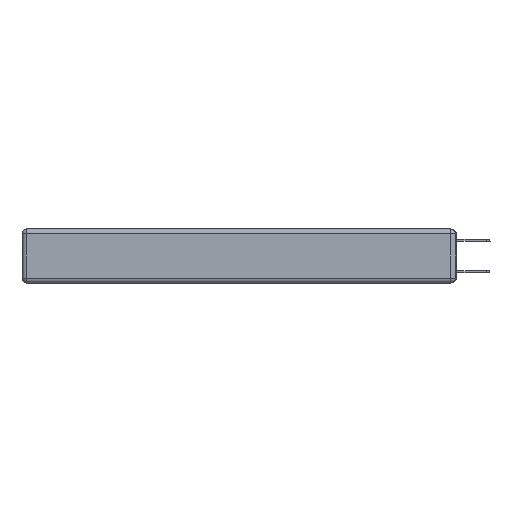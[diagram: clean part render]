
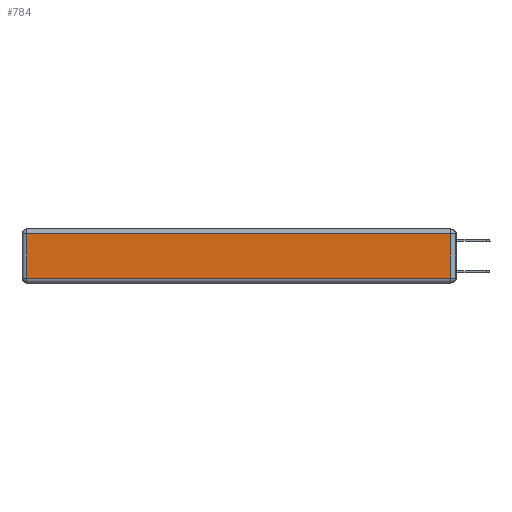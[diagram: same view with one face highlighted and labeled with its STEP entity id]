
A CAD part, left-side view. The second image highlights one B-rep face of the part: STEP entity #784.
In plain terms, the highlighted planar face has unit normal (-1, 0, 0).
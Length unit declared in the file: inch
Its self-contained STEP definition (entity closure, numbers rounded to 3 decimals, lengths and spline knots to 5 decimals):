
#784 = ADVANCED_FACE ( 'NONE', ( #7950 ), #14610, .T. ) ;
#2665 = CARTESIAN_POINT ( 'NONE',  ( 0., 2.72, -0.03 ) ) ;
#5371 = LINE ( 'NONE', #16975, #28543 ) ;
#6753 = DIRECTION ( 'NONE',  ( 0., 0., 1. ) ) ;
#6854 = VERTEX_POINT ( 'NONE', #11180 ) ;
#6976 = CARTESIAN_POINT ( 'NONE',  ( 0., 2.75, -0.03 ) ) ;
#7052 = ORIENTED_EDGE ( 'NONE', *, *, #9930, .T. ) ;
#7124 = LINE ( 'NONE', #6976, #26801 ) ;
#7950 = FACE_OUTER_BOUND ( 'NONE', #23447, .T. ) ;
#8433 = CARTESIAN_POINT ( 'NONE',  ( 0., 0.03, -0.313 ) ) ;
#9315 = ORIENTED_EDGE ( 'NONE', *, *, #19099, .T. ) ;
#9930 = EDGE_CURVE ( 'NONE', #11131, #17355, #5371, .T. ) ;
#10150 = DIRECTION ( 'NONE',  ( 0., 0., -1. ) ) ;
#11091 = ORIENTED_EDGE ( 'NONE', *, *, #26336, .T. ) ;
#11131 = VERTEX_POINT ( 'NONE', #2665 ) ;
#11180 = CARTESIAN_POINT ( 'NONE',  ( 0., 0.03, -0.03 ) ) ;
#12395 = AXIS2_PLACEMENT_3D ( 'NONE', #23473, #19423, #12870 ) ;
#12870 = DIRECTION ( 'NONE',  ( 0., 0., 1. ) ) ;
#13628 = DIRECTION ( 'NONE',  ( 0., 1., 0. ) ) ;
#14610 = PLANE ( 'NONE',  #12395 ) ;
#15661 = DIRECTION ( 'NONE',  ( 0., -1., 0. ) ) ;
#15860 = LINE ( 'NONE', #24742, #25571 ) ;
#15976 = CARTESIAN_POINT ( 'NONE',  ( 0., 2.72, -0.313 ) ) ;
#16975 = CARTESIAN_POINT ( 'NONE',  ( 0., 2.72, -0.343 ) ) ;
#17355 = VERTEX_POINT ( 'NONE', #15976 ) ;
#17975 = LINE ( 'NONE', #24398, #22885 ) ;
#19099 = EDGE_CURVE ( 'NONE', #6854, #11131, #7124, .T. ) ;
#19423 = DIRECTION ( 'NONE',  ( -1., 0., 0. ) ) ;
#22885 = VECTOR ( 'NONE', #15661, 39.37008 ) ;
#23447 = EDGE_LOOP ( 'NONE', ( #28520, #11091, #9315, #7052 ) ) ;
#23473 = CARTESIAN_POINT ( 'NONE',  ( 0., 0., -0.343 ) ) ;
#24398 = CARTESIAN_POINT ( 'NONE',  ( 0., 0., -0.313 ) ) ;
#24742 = CARTESIAN_POINT ( 'NONE',  ( 0., 0.03, -0.343 ) ) ;
#24755 = VERTEX_POINT ( 'NONE', #8433 ) ;
#25571 = VECTOR ( 'NONE', #6753, 39.37008 ) ;
#26336 = EDGE_CURVE ( 'NONE', #24755, #6854, #15860, .T. ) ;
#26655 = EDGE_CURVE ( 'NONE', #17355, #24755, #17975, .T. ) ;
#26801 = VECTOR ( 'NONE', #13628, 39.37008 ) ;
#28520 = ORIENTED_EDGE ( 'NONE', *, *, #26655, .T. ) ;
#28543 = VECTOR ( 'NONE', #10150, 39.37008 ) ;
